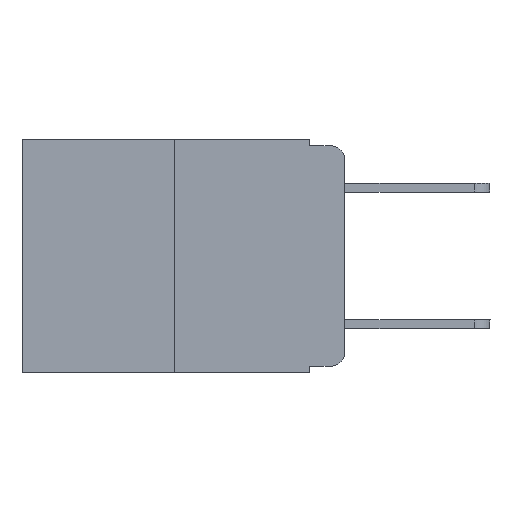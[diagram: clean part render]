
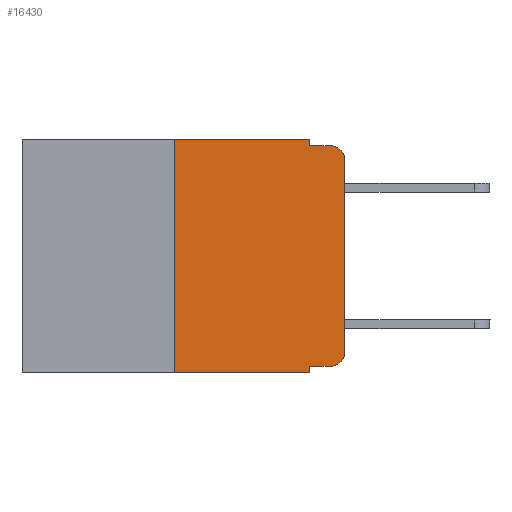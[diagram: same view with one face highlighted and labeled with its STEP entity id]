
A CAD part, left-side view. The second image highlights one B-rep face of the part: STEP entity #16430.
In plain terms, the highlighted planar face has unit normal (-1, 0, 0).
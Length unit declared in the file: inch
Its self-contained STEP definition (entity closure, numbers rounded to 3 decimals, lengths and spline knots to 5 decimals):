
#300 = CARTESIAN_POINT ( 'NONE',  ( 0., 0.02, -0.03 ) ) ;
#555 = ORIENTED_EDGE ( 'NONE', *, *, #4433, .T. ) ;
#634 = CARTESIAN_POINT ( 'NONE',  ( 0., 0.473, 0. ) ) ;
#691 = VERTEX_POINT ( 'NONE', #13472 ) ;
#871 = CIRCLE ( 'NONE', #1240, 0.02 ) ;
#909 = FACE_OUTER_BOUND ( 'NONE', #9299, .T. ) ;
#1240 = AXIS2_PLACEMENT_3D ( 'NONE', #8341, #1801, #16084 ) ;
#1313 = ORIENTED_EDGE ( 'NONE', *, *, #9417, .F. ) ;
#1359 = LINE ( 'NONE', #14520, #10574 ) ;
#1430 = DIRECTION ( 'NONE',  ( 0., -1., 0. ) ) ;
#1459 = EDGE_CURVE ( 'NONE', #9232, #7144, #871, .T. ) ;
#1490 = EDGE_CURVE ( 'NONE', #11844, #8691, #6267, .T. ) ;
#1801 = DIRECTION ( 'NONE',  ( -1., 0., 0. ) ) ;
#2545 = DIRECTION ( 'NONE',  ( 0., 0., 1. ) ) ;
#2549 = AXIS2_PLACEMENT_3D ( 'NONE', #300, #14499, #6719 ) ;
#2947 = ORIENTED_EDGE ( 'NONE', *, *, #5249, .T. ) ;
#3166 = VECTOR ( 'NONE', #9591, 39.37008 ) ;
#3202 = CARTESIAN_POINT ( 'NONE',  ( 0., 0.051, -0.01 ) ) ;
#3489 = LINE ( 'NONE', #9049, #6082 ) ;
#3964 = VECTOR ( 'NONE', #1430, 39.37008 ) ;
#4152 = LINE ( 'NONE', #10266, #3964 ) ;
#4433 = EDGE_CURVE ( 'NONE', #13809, #9232, #4152, .T. ) ;
#4484 = DIRECTION ( 'NONE',  ( 1., 0., 0. ) ) ;
#4570 = VERTEX_POINT ( 'NONE', #9135 ) ;
#4597 = PLANE ( 'NONE',  #6948 ) ;
#4658 = VECTOR ( 'NONE', #5815, 39.37008 ) ;
#4759 = EDGE_CURVE ( 'NONE', #4570, #8904, #6157, .T. ) ;
#5162 = ORIENTED_EDGE ( 'NONE', *, *, #1459, .T. ) ;
#5249 = EDGE_CURVE ( 'NONE', #7144, #691, #16628, .T. ) ;
#5719 = CARTESIAN_POINT ( 'NONE',  ( 0., 0.051, 0. ) ) ;
#5815 = DIRECTION ( 'NONE',  ( 0., -1., 0. ) ) ;
#6057 = CARTESIAN_POINT ( 'NONE',  ( 0., 0.051, -0.343 ) ) ;
#6082 = VECTOR ( 'NONE', #6527, 39.37008 ) ;
#6157 = LINE ( 'NONE', #15927, #12592 ) ;
#6267 = LINE ( 'NONE', #3202, #4658 ) ;
#6527 = DIRECTION ( 'NONE',  ( 0., 0., 1. ) ) ;
#6569 = EDGE_CURVE ( 'NONE', #10553, #4570, #3489, .T. ) ;
#6652 = CARTESIAN_POINT ( 'NONE',  ( 0., 0., -0.313 ) ) ;
#6717 = VECTOR ( 'NONE', #6904, 39.37008 ) ;
#6719 = DIRECTION ( 'NONE',  ( 0., 0., -1. ) ) ;
#6737 = ORIENTED_EDGE ( 'NONE', *, *, #6569, .F. ) ;
#6846 = CARTESIAN_POINT ( 'NONE',  ( 0., 0.473, -0.343 ) ) ;
#6904 = DIRECTION ( 'NONE',  ( 0., -1., 0. ) ) ;
#6948 = AXIS2_PLACEMENT_3D ( 'NONE', #634, #4484, #13913 ) ;
#7063 = CIRCLE ( 'NONE', #2549, 0.02 ) ;
#7144 = VERTEX_POINT ( 'NONE', #6652 ) ;
#7766 = CARTESIAN_POINT ( 'NONE',  ( 0., 0., 0. ) ) ;
#8341 = CARTESIAN_POINT ( 'NONE',  ( 0., 0.02, -0.313 ) ) ;
#8691 = VERTEX_POINT ( 'NONE', #12294 ) ;
#8767 = VERTEX_POINT ( 'NONE', #6057 ) ;
#8785 = CARTESIAN_POINT ( 'NONE',  ( 0., 0.051, -0.333 ) ) ;
#8904 = VERTEX_POINT ( 'NONE', #14793 ) ;
#9049 = CARTESIAN_POINT ( 'NONE',  ( 0., 0.25, 0. ) ) ;
#9135 = CARTESIAN_POINT ( 'NONE',  ( 0., 0.25, 0. ) ) ;
#9203 = ORIENTED_EDGE ( 'NONE', *, *, #15654, .T. ) ;
#9232 = VERTEX_POINT ( 'NONE', #13113 ) ;
#9299 = EDGE_LOOP ( 'NONE', ( #2947, #10313, #14049, #15862, #14560, #6737, #9203, #1313, #555, #5162 ) ) ;
#9417 = EDGE_CURVE ( 'NONE', #13809, #8767, #13853, .T. ) ;
#9591 = DIRECTION ( 'NONE',  ( 0., 0., -1. ) ) ;
#10266 = CARTESIAN_POINT ( 'NONE',  ( 0., 0.051, -0.333 ) ) ;
#10313 = ORIENTED_EDGE ( 'NONE', *, *, #12650, .T. ) ;
#10553 = VERTEX_POINT ( 'NONE', #14531 ) ;
#10574 = VECTOR ( 'NONE', #13065, 39.37008 ) ;
#10868 = DIRECTION ( 'NONE',  ( 0., -1., 0. ) ) ;
#11747 = LINE ( 'NONE', #6846, #6717 ) ;
#11844 = VERTEX_POINT ( 'NONE', #11873 ) ;
#11873 = CARTESIAN_POINT ( 'NONE',  ( 0., 0.051, -0.01 ) ) ;
#12294 = CARTESIAN_POINT ( 'NONE',  ( 0., 0.02, -0.01 ) ) ;
#12592 = VECTOR ( 'NONE', #10868, 39.37008 ) ;
#12650 = EDGE_CURVE ( 'NONE', #691, #8691, #7063, .T. ) ;
#12975 = VECTOR ( 'NONE', #2545, 39.37008 ) ;
#13065 = DIRECTION ( 'NONE',  ( 0., 0., -1. ) ) ;
#13113 = CARTESIAN_POINT ( 'NONE',  ( 0., 0.02, -0.333 ) ) ;
#13472 = CARTESIAN_POINT ( 'NONE',  ( 0., 0., -0.03 ) ) ;
#13809 = VERTEX_POINT ( 'NONE', #8785 ) ;
#13853 = LINE ( 'NONE', #5719, #3166 ) ;
#13913 = DIRECTION ( 'NONE',  ( 0., 0., -1. ) ) ;
#14049 = ORIENTED_EDGE ( 'NONE', *, *, #1490, .F. ) ;
#14499 = DIRECTION ( 'NONE',  ( -1., 0., 0. ) ) ;
#14520 = CARTESIAN_POINT ( 'NONE',  ( 0., 0.051, 0. ) ) ;
#14531 = CARTESIAN_POINT ( 'NONE',  ( 0., 0.25, -0.343 ) ) ;
#14560 = ORIENTED_EDGE ( 'NONE', *, *, #4759, .F. ) ;
#14793 = CARTESIAN_POINT ( 'NONE',  ( 0., 0.051, 0. ) ) ;
#15199 = EDGE_CURVE ( 'NONE', #8904, #11844, #1359, .T. ) ;
#15654 = EDGE_CURVE ( 'NONE', #10553, #8767, #11747, .T. ) ;
#15862 = ORIENTED_EDGE ( 'NONE', *, *, #15199, .F. ) ;
#15927 = CARTESIAN_POINT ( 'NONE',  ( 0., 0.473, 0. ) ) ;
#16084 = DIRECTION ( 'NONE',  ( 0., 0., -1. ) ) ;
#16430 = ADVANCED_FACE ( 'NONE', ( #909 ), #4597, .F. ) ;
#16628 = LINE ( 'NONE', #7766, #12975 ) ;
